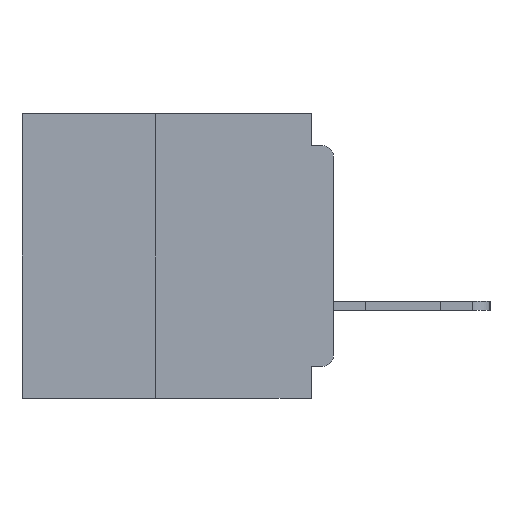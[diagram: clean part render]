
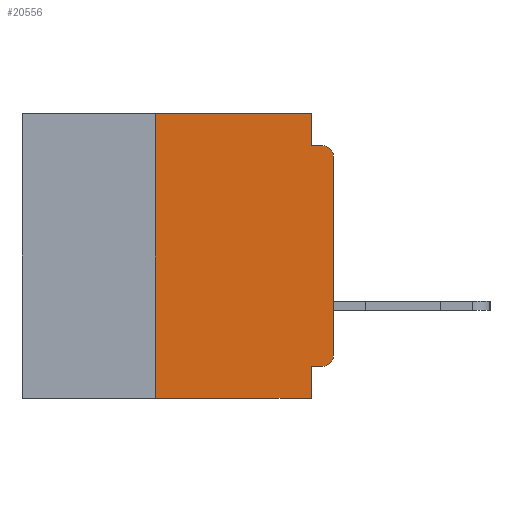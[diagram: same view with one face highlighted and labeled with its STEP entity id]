
A CAD part, left-side view. The second image highlights one B-rep face of the part: STEP entity #20556.
In plain terms, the highlighted planar face has unit normal (-1, 0, 0).
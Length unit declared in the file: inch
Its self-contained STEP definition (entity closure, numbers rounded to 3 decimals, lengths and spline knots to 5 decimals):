
#405 = DIRECTION ( 'NONE',  ( 0., -1., 0. ) ) ;
#844 = CARTESIAN_POINT ( 'NONE',  ( 0., 0.437, 0. ) ) ;
#875 = CARTESIAN_POINT ( 'NONE',  ( 0., 0., -0.06 ) ) ;
#899 = CARTESIAN_POINT ( 'NONE',  ( 0., 0.031, 0. ) ) ;
#1580 = CARTESIAN_POINT ( 'NONE',  ( 0., 0.015, -0.045 ) ) ;
#1767 = VERTEX_POINT ( 'NONE', #4002 ) ;
#1808 = DIRECTION ( 'NONE',  ( 0., 1., 0. ) ) ;
#2057 = EDGE_CURVE ( 'NONE', #30385, #12217, #4771, .T. ) ;
#3602 = EDGE_CURVE ( 'NONE', #18618, #36001, #28731, .T. ) ;
#3818 = CARTESIAN_POINT ( 'NONE',  ( 0., 0.015, -0.355 ) ) ;
#4002 = CARTESIAN_POINT ( 'NONE',  ( 0., 0.25, -0.4 ) ) ;
#4183 = DIRECTION ( 'NONE',  ( 0., -1., 0. ) ) ;
#4651 = DIRECTION ( 'NONE',  ( -1., 0., 0. ) ) ;
#4699 = LINE ( 'NONE', #27160, #13608 ) ;
#4771 = LINE ( 'NONE', #12608, #39262 ) ;
#6703 = AXIS2_PLACEMENT_3D ( 'NONE', #24747, #4651, #28073 ) ;
#7881 = EDGE_CURVE ( 'NONE', #15873, #30385, #29122, .T. ) ;
#8109 = AXIS2_PLACEMENT_3D ( 'NONE', #18317, #41563, #21675 ) ;
#9868 = EDGE_CURVE ( 'NONE', #12217, #36899, #31120, .T. ) ;
#12217 = VERTEX_POINT ( 'NONE', #34430 ) ;
#12433 = ORIENTED_EDGE ( 'NONE', *, *, #15710, .F. ) ;
#12445 = ORIENTED_EDGE ( 'NONE', *, *, #32499, .T. ) ;
#12608 = CARTESIAN_POINT ( 'NONE',  ( 0., 0.031, 0. ) ) ;
#12647 = VECTOR ( 'NONE', #1808, 39.37008 ) ;
#12756 = DIRECTION ( 'NONE',  ( 0., 0., -1. ) ) ;
#13608 = VECTOR ( 'NONE', #405, 39.37008 ) ;
#14335 = VECTOR ( 'NONE', #42114, 39.37008 ) ;
#14674 = DIRECTION ( 'NONE',  ( 0., 0., 1. ) ) ;
#15114 = CARTESIAN_POINT ( 'NONE',  ( 0., 0., 0. ) ) ;
#15518 = ORIENTED_EDGE ( 'NONE', *, *, #2057, .F. ) ;
#15710 = EDGE_CURVE ( 'NONE', #30324, #30278, #39276, .T. ) ;
#15873 = VERTEX_POINT ( 'NONE', #35860 ) ;
#16463 = EDGE_LOOP ( 'NONE', ( #38173, #12445, #35287, #15518, #22312, #35796, #26771, #35276, #12433, #25561 ) ) ;
#16800 = CARTESIAN_POINT ( 'NONE',  ( 0., 0.25, -0.4 ) ) ;
#17084 = AXIS2_PLACEMENT_3D ( 'NONE', #38606, #21865, #22011 ) ;
#18317 = CARTESIAN_POINT ( 'NONE',  ( 0., 0.015, -0.06 ) ) ;
#18477 = CIRCLE ( 'NONE', #6703, 0.015 ) ;
#18496 = CARTESIAN_POINT ( 'NONE',  ( 0., 0., -0.355 ) ) ;
#18618 = VERTEX_POINT ( 'NONE', #34085 ) ;
#18799 = VECTOR ( 'NONE', #14674, 39.37008 ) ;
#18866 = CARTESIAN_POINT ( 'NONE',  ( 0., 0., -0.045 ) ) ;
#19732 = CARTESIAN_POINT ( 'NONE',  ( 0., 0.031, -0.4 ) ) ;
#20235 = VECTOR ( 'NONE', #4183, 39.37008 ) ;
#20556 = ADVANCED_FACE ( 'NONE', ( #21427 ), #41899, .F. ) ;
#20903 = VECTOR ( 'NONE', #23371, 39.37008 ) ;
#21427 = FACE_OUTER_BOUND ( 'NONE', #16463, .T. ) ;
#21452 = EDGE_CURVE ( 'NONE', #1767, #15873, #41694, .T. ) ;
#21675 = DIRECTION ( 'NONE',  ( 0., 0., -1. ) ) ;
#21865 = DIRECTION ( 'NONE',  ( 1., 0., 0. ) ) ;
#22011 = DIRECTION ( 'NONE',  ( 0., 0., -1. ) ) ;
#22310 = LINE ( 'NONE', #19732, #38975 ) ;
#22312 = ORIENTED_EDGE ( 'NONE', *, *, #7881, .F. ) ;
#23371 = DIRECTION ( 'NONE',  ( 0., 0., 1. ) ) ;
#24325 = EDGE_CURVE ( 'NONE', #30278, #39132, #22310, .T. ) ;
#24747 = CARTESIAN_POINT ( 'NONE',  ( 0., 0.015, -0.34 ) ) ;
#25561 = ORIENTED_EDGE ( 'NONE', *, *, #41748, .T. ) ;
#26279 = CIRCLE ( 'NONE', #8109, 0.015 ) ;
#26771 = ORIENTED_EDGE ( 'NONE', *, *, #42961, .T. ) ;
#26965 = CARTESIAN_POINT ( 'NONE',  ( 0., 0.031, -0.355 ) ) ;
#27160 = CARTESIAN_POINT ( 'NONE',  ( 0., 0.437, -0.4 ) ) ;
#28073 = DIRECTION ( 'NONE',  ( 0., 0., -1. ) ) ;
#28731 = LINE ( 'NONE', #15114, #18799 ) ;
#29122 = LINE ( 'NONE', #844, #20235 ) ;
#30278 = VERTEX_POINT ( 'NONE', #26965 ) ;
#30324 = VERTEX_POINT ( 'NONE', #3818 ) ;
#30385 = VERTEX_POINT ( 'NONE', #899 ) ;
#31120 = LINE ( 'NONE', #18866, #14335 ) ;
#32499 = EDGE_CURVE ( 'NONE', #36001, #36899, #26279, .T. ) ;
#34085 = CARTESIAN_POINT ( 'NONE',  ( 0., 0., -0.34 ) ) ;
#34430 = CARTESIAN_POINT ( 'NONE',  ( 0., 0.031, -0.045 ) ) ;
#35276 = ORIENTED_EDGE ( 'NONE', *, *, #24325, .F. ) ;
#35287 = ORIENTED_EDGE ( 'NONE', *, *, #9868, .F. ) ;
#35796 = ORIENTED_EDGE ( 'NONE', *, *, #21452, .F. ) ;
#35860 = CARTESIAN_POINT ( 'NONE',  ( 0., 0.25, 0. ) ) ;
#36001 = VERTEX_POINT ( 'NONE', #875 ) ;
#36899 = VERTEX_POINT ( 'NONE', #1580 ) ;
#38173 = ORIENTED_EDGE ( 'NONE', *, *, #3602, .T. ) ;
#38606 = CARTESIAN_POINT ( 'NONE',  ( 0., 0.437, 0. ) ) ;
#38975 = VECTOR ( 'NONE', #42667, 39.37008 ) ;
#39132 = VERTEX_POINT ( 'NONE', #40748 ) ;
#39262 = VECTOR ( 'NONE', #12756, 39.37008 ) ;
#39276 = LINE ( 'NONE', #18496, #12647 ) ;
#40748 = CARTESIAN_POINT ( 'NONE',  ( 0., 0.031, -0.4 ) ) ;
#41563 = DIRECTION ( 'NONE',  ( -1., 0., 0. ) ) ;
#41694 = LINE ( 'NONE', #16800, #20903 ) ;
#41748 = EDGE_CURVE ( 'NONE', #30324, #18618, #18477, .T. ) ;
#41899 = PLANE ( 'NONE',  #17084 ) ;
#42114 = DIRECTION ( 'NONE',  ( 0., -1., 0. ) ) ;
#42667 = DIRECTION ( 'NONE',  ( 0., 0., -1. ) ) ;
#42961 = EDGE_CURVE ( 'NONE', #1767, #39132, #4699, .T. ) ;
